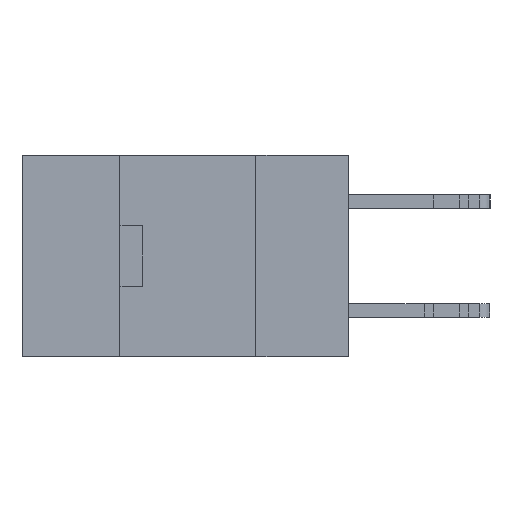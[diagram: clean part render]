
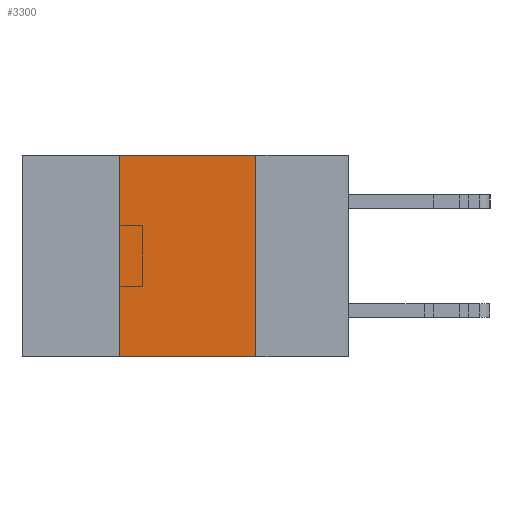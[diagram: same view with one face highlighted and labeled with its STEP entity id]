
A CAD part, left-side view. The second image highlights one B-rep face of the part: STEP entity #3300.
In plain terms, the highlighted planar face has unit normal (-1, 0, 0).
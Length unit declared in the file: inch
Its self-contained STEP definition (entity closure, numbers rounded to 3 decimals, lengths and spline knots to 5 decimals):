
#46 = CARTESIAN_POINT ( 'NONE',  ( 0., 0.42, -0.37 ) ) ;
#318 = DIRECTION ( 'NONE',  ( 0., -1., 0. ) ) ;
#1477 = EDGE_LOOP ( 'NONE', ( #23408, #16473, #6247, #14757 ) ) ;
#3215 = VERTEX_POINT ( 'NONE', #17157 ) ;
#3300 = ADVANCED_FACE ( 'NONE', ( #6004 ), #11277, .F. ) ;
#4709 = CARTESIAN_POINT ( 'NONE',  ( 0., 0.6, 0. ) ) ;
#6004 = FACE_OUTER_BOUND ( 'NONE', #1477, .T. ) ;
#6247 = ORIENTED_EDGE ( 'NONE', *, *, #24930, .F. ) ;
#8452 = DIRECTION ( 'NONE',  ( 0., -1., 0. ) ) ;
#8721 = DIRECTION ( 'NONE',  ( 0., 0., -1. ) ) ;
#10513 = VECTOR ( 'NONE', #318, 39.37008 ) ;
#10910 = LINE ( 'NONE', #13339, #10513 ) ;
#10920 = LINE ( 'NONE', #46, #19271 ) ;
#11217 = AXIS2_PLACEMENT_3D ( 'NONE', #4709, #19766, #8721 ) ;
#11277 = PLANE ( 'NONE',  #11217 ) ;
#12243 = VECTOR ( 'NONE', #8452, 39.37008 ) ;
#12464 = CARTESIAN_POINT ( 'NONE',  ( 0., 0.6, 0. ) ) ;
#12821 = CARTESIAN_POINT ( 'NONE',  ( 0., 0.17, -0.37 ) ) ;
#13296 = CARTESIAN_POINT ( 'NONE',  ( 0., 0.42, -0.37 ) ) ;
#13339 = CARTESIAN_POINT ( 'NONE',  ( 0., 0.6, -0.37 ) ) ;
#14757 = ORIENTED_EDGE ( 'NONE', *, *, #23534, .T. ) ;
#15894 = VERTEX_POINT ( 'NONE', #13296 ) ;
#16033 = VECTOR ( 'NONE', #21593, 39.37008 ) ;
#16473 = ORIENTED_EDGE ( 'NONE', *, *, #19412, .F. ) ;
#17157 = CARTESIAN_POINT ( 'NONE',  ( 0., 0.42, 0. ) ) ;
#19271 = VECTOR ( 'NONE', #26567, 39.37008 ) ;
#19412 = EDGE_CURVE ( 'NONE', #3215, #22962, #26108, .T. ) ;
#19766 = DIRECTION ( 'NONE',  ( 1., 0., 0. ) ) ;
#19994 = CARTESIAN_POINT ( 'NONE',  ( 0., 0.17, 0. ) ) ;
#21306 = LINE ( 'NONE', #12821, #16033 ) ;
#21593 = DIRECTION ( 'NONE',  ( 0., 0., -1. ) ) ;
#22851 = VERTEX_POINT ( 'NONE', #25611 ) ;
#22962 = VERTEX_POINT ( 'NONE', #19994 ) ;
#23408 = ORIENTED_EDGE ( 'NONE', *, *, #24286, .F. ) ;
#23534 = EDGE_CURVE ( 'NONE', #15894, #22851, #10910, .T. ) ;
#24286 = EDGE_CURVE ( 'NONE', #22962, #22851, #21306, .T. ) ;
#24930 = EDGE_CURVE ( 'NONE', #15894, #3215, #10920, .T. ) ;
#25611 = CARTESIAN_POINT ( 'NONE',  ( 0., 0.17, -0.37 ) ) ;
#26108 = LINE ( 'NONE', #12464, #12243 ) ;
#26567 = DIRECTION ( 'NONE',  ( 0., 0., 1. ) ) ;
